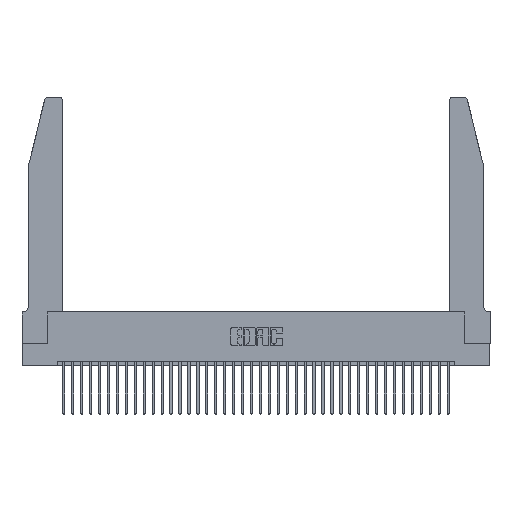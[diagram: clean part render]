
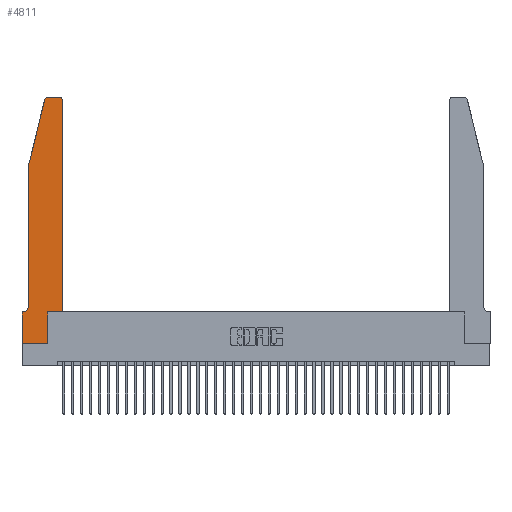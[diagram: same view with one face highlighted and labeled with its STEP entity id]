
A CAD part, top view. The second image highlights one B-rep face of the part: STEP entity #4811.
In plain terms, the highlighted planar face has unit normal (0, 0, 1).
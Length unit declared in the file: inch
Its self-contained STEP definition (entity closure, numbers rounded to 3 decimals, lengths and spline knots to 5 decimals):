
#779 = ORIENTED_EDGE ( 'NONE', *, *, #5313, .T. ) ;
#1761 = DIRECTION ( 'NONE',  ( -1., 0., 0. ) ) ;
#1943 = DIRECTION ( 'NONE',  ( 0., -1., 0. ) ) ;
#2089 = CARTESIAN_POINT ( 'NONE',  ( 0.4205, 2.72, 0.37 ) ) ;
#2309 = VECTOR ( 'NONE', #31922, 39.37008 ) ;
#2530 = EDGE_LOOP ( 'NONE', ( #6741, #11579, #5441, #27834, #22938, #34212, #38704, #25266, #779, #10642, #13198, #4268 ) ) ;
#2782 = DIRECTION ( 'NONE',  ( 0., 0., 1. ) ) ;
#2880 = CARTESIAN_POINT ( 'NONE',  ( 0.4205, 2.75, 0.37 ) ) ;
#3685 = CARTESIAN_POINT ( 'NONE',  ( 0.284, 2.72, 0.37 ) ) ;
#4175 = CARTESIAN_POINT ( 'NONE',  ( 0.25487, 2.72718, 0.37 ) ) ;
#4268 = ORIENTED_EDGE ( 'NONE', *, *, #20853, .T. ) ;
#4316 = DIRECTION ( 'NONE',  ( 1., 0., 0. ) ) ;
#4767 = CARTESIAN_POINT ( 'NONE',  ( 0.2605, 2.75, 0.37 ) ) ;
#4811 = ADVANCED_FACE ( 'NONE', ( #27821 ), #14747, .T. ) ;
#4895 = DIRECTION ( 'NONE',  ( -1., 0., 0. ) ) ;
#5313 = EDGE_CURVE ( 'NONE', #35864, #13727, #26348, .T. ) ;
#5398 = DIRECTION ( 'NONE',  ( 1., 0., 0. ) ) ;
#5441 = ORIENTED_EDGE ( 'NONE', *, *, #18921, .T. ) ;
#5844 = CARTESIAN_POINT ( 'NONE',  ( 0., 0.35, 0.37 ) ) ;
#5905 = VERTEX_POINT ( 'NONE', #2880 ) ;
#5946 = DIRECTION ( 'NONE',  ( 1., 0., 0. ) ) ;
#5964 = VERTEX_POINT ( 'NONE', #4175 ) ;
#6042 = LINE ( 'NONE', #4767, #22510 ) ;
#6741 = ORIENTED_EDGE ( 'NONE', *, *, #8110, .T. ) ;
#7685 = EDGE_CURVE ( 'NONE', #10186, #35864, #36723, .T. ) ;
#7903 = CARTESIAN_POINT ( 'NONE',  ( 0.2865, 0., 0.37 ) ) ;
#8110 = EDGE_CURVE ( 'NONE', #5905, #28819, #6042, .T. ) ;
#8340 = EDGE_CURVE ( 'NONE', #26510, #22644, #26276, .T. ) ;
#8394 = VERTEX_POINT ( 'NONE', #26879 ) ;
#8654 = CARTESIAN_POINT ( 'NONE',  ( 0.0755, 2., 0.37 ) ) ;
#8697 = LINE ( 'NONE', #16939, #26588 ) ;
#8835 = CARTESIAN_POINT ( 'NONE',  ( 0., 0., 0.37 ) ) ;
#9841 = CARTESIAN_POINT ( 'NONE',  ( 0.4505, 0.35, 0.37 ) ) ;
#10137 = VECTOR ( 'NONE', #4316, 39.37008 ) ;
#10186 = VERTEX_POINT ( 'NONE', #8835 ) ;
#10458 = CARTESIAN_POINT ( 'NONE',  ( 0.0755, 0.35, 0.37 ) ) ;
#10642 = ORIENTED_EDGE ( 'NONE', *, *, #36446, .T. ) ;
#11225 = EDGE_CURVE ( 'NONE', #17767, #10186, #20308, .T. ) ;
#11402 = AXIS2_PLACEMENT_3D ( 'NONE', #20805, #2782, #5946 ) ;
#11579 = ORIENTED_EDGE ( 'NONE', *, *, #34159, .T. ) ;
#13084 = EDGE_CURVE ( 'NONE', #38736, #34972, #18040, .T. ) ;
#13198 = ORIENTED_EDGE ( 'NONE', *, *, #8340, .T. ) ;
#13570 = DIRECTION ( 'NONE',  ( 0., 0., -1. ) ) ;
#13727 = VERTEX_POINT ( 'NONE', #22733 ) ;
#14390 = DIRECTION ( 'NONE',  ( 0., 1., 0. ) ) ;
#14558 = CARTESIAN_POINT ( 'NONE',  ( 0.4505, 2.72, 0.37 ) ) ;
#14747 = PLANE ( 'NONE',  #11402 ) ;
#16939 = CARTESIAN_POINT ( 'NONE',  ( 0.0755, 2., 0.37 ) ) ;
#17767 = VERTEX_POINT ( 'NONE', #5844 ) ;
#18040 = CIRCLE ( 'NONE', #23138, 0.07 ) ;
#18650 = CARTESIAN_POINT ( 'NONE',  ( 0.0055, 0.35, 0.37 ) ) ;
#18921 = EDGE_CURVE ( 'NONE', #5964, #8394, #32203, .T. ) ;
#18970 = DIRECTION ( 'NONE',  ( 0., 0., 1. ) ) ;
#20308 = LINE ( 'NONE', #31556, #23584 ) ;
#20330 = CARTESIAN_POINT ( 'NONE',  ( 0.0755, 0.42, 0.37 ) ) ;
#20700 = CARTESIAN_POINT ( 'NONE',  ( 0.4505, 0.35, 0.37 ) ) ;
#20805 = CARTESIAN_POINT ( 'NONE',  ( 0., 0.35, 0.37 ) ) ;
#20853 = EDGE_CURVE ( 'NONE', #22644, #5905, #22109, .T. ) ;
#22109 = CIRCLE ( 'NONE', #24648, 0.03 ) ;
#22510 = VECTOR ( 'NONE', #1761, 39.37008 ) ;
#22644 = VERTEX_POINT ( 'NONE', #14558 ) ;
#22733 = CARTESIAN_POINT ( 'NONE',  ( 0.2865, 0.35, 0.37 ) ) ;
#22840 = LINE ( 'NONE', #9841, #10137 ) ;
#22938 = ORIENTED_EDGE ( 'NONE', *, *, #13084, .T. ) ;
#23138 = AXIS2_PLACEMENT_3D ( 'NONE', #34906, #13570, #4895 ) ;
#23584 = VECTOR ( 'NONE', #28366, 39.37008 ) ;
#24468 = DIRECTION ( 'NONE',  ( 1., 0., 0. ) ) ;
#24648 = AXIS2_PLACEMENT_3D ( 'NONE', #2089, #26150, #32232 ) ;
#24904 = AXIS2_PLACEMENT_3D ( 'NONE', #3685, #18970, #24468 ) ;
#25266 = ORIENTED_EDGE ( 'NONE', *, *, #7685, .T. ) ;
#25764 = VECTOR ( 'NONE', #14390, 39.37008 ) ;
#26150 = DIRECTION ( 'NONE',  ( 0., 0., 1. ) ) ;
#26276 = LINE ( 'NONE', #20700, #25764 ) ;
#26348 = LINE ( 'NONE', #33595, #28228 ) ;
#26510 = VERTEX_POINT ( 'NONE', #35454 ) ;
#26588 = VECTOR ( 'NONE', #1943, 39.37008 ) ;
#26696 = CARTESIAN_POINT ( 'NONE',  ( 0., 0., 0.37 ) ) ;
#26879 = CARTESIAN_POINT ( 'NONE',  ( 0.0755, 2., 0.37 ) ) ;
#27821 = FACE_OUTER_BOUND ( 'NONE', #2530, .T. ) ;
#27834 = ORIENTED_EDGE ( 'NONE', *, *, #36665, .T. ) ;
#28228 = VECTOR ( 'NONE', #36118, 39.37008 ) ;
#28366 = DIRECTION ( 'NONE',  ( 0., -1., 0. ) ) ;
#28819 = VERTEX_POINT ( 'NONE', #31227 ) ;
#29167 = VECTOR ( 'NONE', #5398, 39.37008 ) ;
#30442 = EDGE_CURVE ( 'NONE', #34972, #17767, #37616, .T. ) ;
#31227 = CARTESIAN_POINT ( 'NONE',  ( 0.284, 2.75, 0.37 ) ) ;
#31556 = CARTESIAN_POINT ( 'NONE',  ( 0., 0., 0.37 ) ) ;
#31922 = DIRECTION ( 'NONE',  ( -1., 0., 0. ) ) ;
#32203 = LINE ( 'NONE', #8654, #33149 ) ;
#32232 = DIRECTION ( 'NONE',  ( 1., 0., 0. ) ) ;
#32626 = DIRECTION ( 'NONE',  ( -0.239, -0.971, 0. ) ) ;
#33149 = VECTOR ( 'NONE', #32626, 39.37008 ) ;
#33595 = CARTESIAN_POINT ( 'NONE',  ( 0.2865, 0.35, 0.37 ) ) ;
#34159 = EDGE_CURVE ( 'NONE', #28819, #5964, #35783, .T. ) ;
#34212 = ORIENTED_EDGE ( 'NONE', *, *, #30442, .T. ) ;
#34906 = CARTESIAN_POINT ( 'NONE',  ( 0.0055, 0.42, 0.37 ) ) ;
#34972 = VERTEX_POINT ( 'NONE', #18650 ) ;
#35454 = CARTESIAN_POINT ( 'NONE',  ( 0.4505, 0.35, 0.37 ) ) ;
#35783 = CIRCLE ( 'NONE', #24904, 0.03 ) ;
#35864 = VERTEX_POINT ( 'NONE', #7903 ) ;
#36118 = DIRECTION ( 'NONE',  ( 0., 1., 0. ) ) ;
#36446 = EDGE_CURVE ( 'NONE', #13727, #26510, #22840, .T. ) ;
#36665 = EDGE_CURVE ( 'NONE', #8394, #38736, #8697, .T. ) ;
#36723 = LINE ( 'NONE', #26696, #29167 ) ;
#37616 = LINE ( 'NONE', #10458, #2309 ) ;
#38704 = ORIENTED_EDGE ( 'NONE', *, *, #11225, .T. ) ;
#38736 = VERTEX_POINT ( 'NONE', #20330 ) ;
